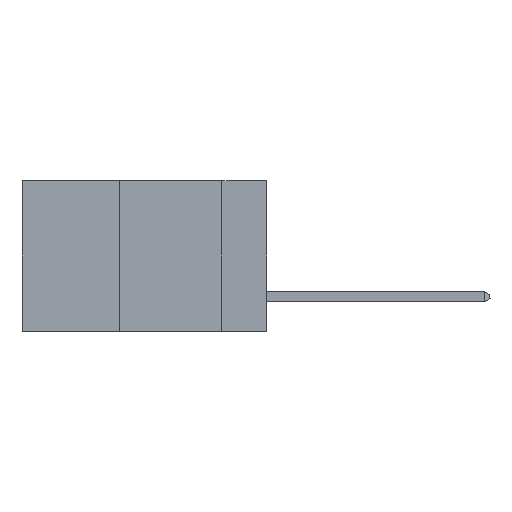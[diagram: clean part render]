
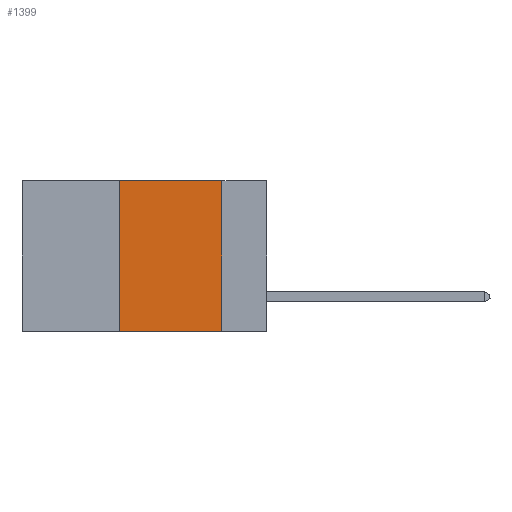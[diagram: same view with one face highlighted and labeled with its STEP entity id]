
A CAD part, left-side view. The second image highlights one B-rep face of the part: STEP entity #1399.
In plain terms, the highlighted planar face has unit normal (-1, 0, 0).
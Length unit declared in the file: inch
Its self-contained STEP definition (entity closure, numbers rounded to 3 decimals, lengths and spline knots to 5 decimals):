
#373 = EDGE_CURVE ( 'NONE', #8277, #5019, #7644, .T. ) ;
#750 = CARTESIAN_POINT ( 'NONE',  ( 0., 0.11, 0. ) ) ;
#1282 = CARTESIAN_POINT ( 'NONE',  ( 0., 0.6, 0. ) ) ;
#1399 = ADVANCED_FACE ( 'NONE', ( #5155 ), #6382, .F. ) ;
#1425 = LINE ( 'NONE', #8274, #5804 ) ;
#1460 = ORIENTED_EDGE ( 'NONE', *, *, #2857, .F. ) ;
#1985 = DIRECTION ( 'NONE',  ( 1., 0., 0. ) ) ;
#2074 = DIRECTION ( 'NONE',  ( 0., -1., 0. ) ) ;
#2183 = CARTESIAN_POINT ( 'NONE',  ( 0., 0.6, -0.37 ) ) ;
#2497 = EDGE_LOOP ( 'NONE', ( #2743, #1460, #11170, #4251 ) ) ;
#2743 = ORIENTED_EDGE ( 'NONE', *, *, #373, .F. ) ;
#2857 = EDGE_CURVE ( 'NONE', #10518, #8277, #6215, .T. ) ;
#2882 = DIRECTION ( 'NONE',  ( 0., 0., 1. ) ) ;
#3196 = EDGE_CURVE ( 'NONE', #11058, #10518, #1425, .T. ) ;
#3425 = VECTOR ( 'NONE', #5622, 39.37008 ) ;
#3714 = LINE ( 'NONE', #2183, #3425 ) ;
#4002 = AXIS2_PLACEMENT_3D ( 'NONE', #4557, #1985, #9843 ) ;
#4251 = ORIENTED_EDGE ( 'NONE', *, *, #11019, .T. ) ;
#4557 = CARTESIAN_POINT ( 'NONE',  ( 0., 0.6, 0. ) ) ;
#4769 = VECTOR ( 'NONE', #7730, 39.37008 ) ;
#5019 = VERTEX_POINT ( 'NONE', #6045 ) ;
#5155 = FACE_OUTER_BOUND ( 'NONE', #2497, .T. ) ;
#5622 = DIRECTION ( 'NONE',  ( 0., -1., 0. ) ) ;
#5804 = VECTOR ( 'NONE', #2882, 39.37008 ) ;
#6045 = CARTESIAN_POINT ( 'NONE',  ( 0., 0.11, -0.37 ) ) ;
#6215 = LINE ( 'NONE', #1282, #8276 ) ;
#6382 = PLANE ( 'NONE',  #4002 ) ;
#7442 = CARTESIAN_POINT ( 'NONE',  ( 0., 0.36, -0.37 ) ) ;
#7644 = LINE ( 'NONE', #750, #4769 ) ;
#7730 = DIRECTION ( 'NONE',  ( 0., 0., -1. ) ) ;
#8274 = CARTESIAN_POINT ( 'NONE',  ( 0., 0.36, 0. ) ) ;
#8276 = VECTOR ( 'NONE', #2074, 39.37008 ) ;
#8277 = VERTEX_POINT ( 'NONE', #10845 ) ;
#8823 = CARTESIAN_POINT ( 'NONE',  ( 0., 0.36, 0. ) ) ;
#9843 = DIRECTION ( 'NONE',  ( 0., 0., -1. ) ) ;
#10518 = VERTEX_POINT ( 'NONE', #8823 ) ;
#10845 = CARTESIAN_POINT ( 'NONE',  ( 0., 0.11, 0. ) ) ;
#11019 = EDGE_CURVE ( 'NONE', #11058, #5019, #3714, .T. ) ;
#11058 = VERTEX_POINT ( 'NONE', #7442 ) ;
#11170 = ORIENTED_EDGE ( 'NONE', *, *, #3196, .F. ) ;
